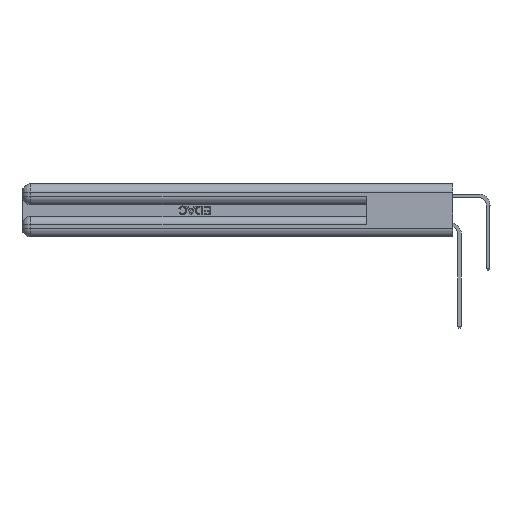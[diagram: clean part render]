
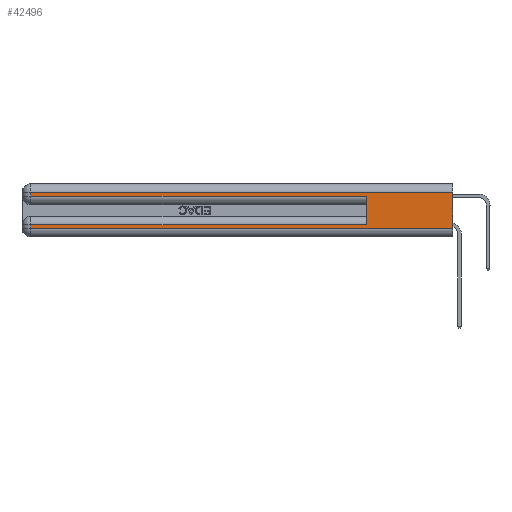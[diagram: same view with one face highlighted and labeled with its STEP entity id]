
A CAD part, left-side view. The second image highlights one B-rep face of the part: STEP entity #42496.
In plain terms, the highlighted planar face has unit normal (-1, 0, 0).
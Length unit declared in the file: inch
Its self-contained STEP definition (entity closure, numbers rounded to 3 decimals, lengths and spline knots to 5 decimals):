
#963 = LINE ( 'NONE', #32042, #27779 ) ;
#1051 = DIRECTION ( 'NONE',  ( 0., 0., -1. ) ) ;
#1064 = EDGE_CURVE ( 'NONE', #27194, #36507, #5275, .T. ) ;
#2364 = DIRECTION ( 'NONE',  ( 0., -1., 0. ) ) ;
#4359 = VERTEX_POINT ( 'NONE', #26455 ) ;
#5062 = CARTESIAN_POINT ( 'NONE',  ( 0., 2.94, 0.085 ) ) ;
#5275 = LINE ( 'NONE', #9818, #41072 ) ;
#5987 = EDGE_CURVE ( 'NONE', #21244, #41450, #963, .T. ) ;
#6390 = CARTESIAN_POINT ( 'NONE',  ( 0., 0., 0.37 ) ) ;
#7752 = VECTOR ( 'NONE', #43807, 39.37008 ) ;
#9786 = EDGE_CURVE ( 'NONE', #21244, #41560, #35603, .T. ) ;
#9818 = CARTESIAN_POINT ( 'NONE',  ( 0., 0., 0.285 ) ) ;
#12184 = ORIENTED_EDGE ( 'NONE', *, *, #14761, .T. ) ;
#12547 = VECTOR ( 'NONE', #1051, 39.37008 ) ;
#13291 = DIRECTION ( 'NONE',  ( 0., -1., 0. ) ) ;
#13956 = DIRECTION ( 'NONE',  ( 0., 0., 1. ) ) ;
#14229 = VECTOR ( 'NONE', #21004, 39.37008 ) ;
#14493 = EDGE_CURVE ( 'NONE', #41450, #27194, #43511, .T. ) ;
#14761 = EDGE_CURVE ( 'NONE', #4359, #32286, #22412, .T. ) ;
#15441 = EDGE_CURVE ( 'NONE', #32286, #34976, #23994, .T. ) ;
#15827 = ORIENTED_EDGE ( 'NONE', *, *, #40106, .T. ) ;
#16718 = DIRECTION ( 'NONE',  ( 0., 0., -1. ) ) ;
#20471 = LINE ( 'NONE', #34735, #28609 ) ;
#20824 = DIRECTION ( 'NONE',  ( 1., 0., 0. ) ) ;
#20885 = CARTESIAN_POINT ( 'NONE',  ( 0., 0.6, 0.285 ) ) ;
#21004 = DIRECTION ( 'NONE',  ( 0., 1., 0. ) ) ;
#21137 = EDGE_CURVE ( 'NONE', #4359, #36507, #20471, .T. ) ;
#21244 = VERTEX_POINT ( 'NONE', #31018 ) ;
#21519 = LINE ( 'NONE', #23303, #30763 ) ;
#21730 = CARTESIAN_POINT ( 'NONE',  ( 0., 0., 0.085 ) ) ;
#22120 = ORIENTED_EDGE ( 'NONE', *, *, #1064, .T. ) ;
#22412 = LINE ( 'NONE', #21730, #14229 ) ;
#23303 = CARTESIAN_POINT ( 'NONE',  ( 0., 0., 0.06 ) ) ;
#23689 = ORIENTED_EDGE ( 'NONE', *, *, #21137, .F. ) ;
#23994 = LINE ( 'NONE', #25380, #12547 ) ;
#25380 = CARTESIAN_POINT ( 'NONE',  ( 0., 2.94, 0.37 ) ) ;
#26134 = ORIENTED_EDGE ( 'NONE', *, *, #9786, .F. ) ;
#26455 = CARTESIAN_POINT ( 'NONE',  ( 0., 0.6, 0.085 ) ) ;
#27194 = VERTEX_POINT ( 'NONE', #33092 ) ;
#27297 = FACE_OUTER_BOUND ( 'NONE', #32736, .T. ) ;
#27779 = VECTOR ( 'NONE', #38953, 39.37008 ) ;
#28498 = AXIS2_PLACEMENT_3D ( 'NONE', #41518, #20824, #44955 ) ;
#28609 = VECTOR ( 'NONE', #13956, 39.37008 ) ;
#30123 = CARTESIAN_POINT ( 'NONE',  ( 0., 2.94, 0.37 ) ) ;
#30154 = ORIENTED_EDGE ( 'NONE', *, *, #14493, .T. ) ;
#30763 = VECTOR ( 'NONE', #2364, 39.37008 ) ;
#31018 = CARTESIAN_POINT ( 'NONE',  ( 0., 0., 0.31 ) ) ;
#31206 = CARTESIAN_POINT ( 'NONE',  ( 0., 2.94, 0.31 ) ) ;
#32042 = CARTESIAN_POINT ( 'NONE',  ( 0., 0., 0.31 ) ) ;
#32286 = VERTEX_POINT ( 'NONE', #5062 ) ;
#32736 = EDGE_LOOP ( 'NONE', ( #26134, #41705, #30154, #22120, #23689, #12184, #39008, #15827 ) ) ;
#33092 = CARTESIAN_POINT ( 'NONE',  ( 0., 2.94, 0.285 ) ) ;
#34529 = VECTOR ( 'NONE', #16718, 39.37008 ) ;
#34735 = CARTESIAN_POINT ( 'NONE',  ( 0., 0.6, 0.145 ) ) ;
#34976 = VERTEX_POINT ( 'NONE', #37746 ) ;
#35098 = CARTESIAN_POINT ( 'NONE',  ( 0., 0., 0.06 ) ) ;
#35603 = LINE ( 'NONE', #6390, #34529 ) ;
#36507 = VERTEX_POINT ( 'NONE', #20885 ) ;
#37746 = CARTESIAN_POINT ( 'NONE',  ( 0., 2.94, 0.06 ) ) ;
#38953 = DIRECTION ( 'NONE',  ( 0., 1., 0. ) ) ;
#39008 = ORIENTED_EDGE ( 'NONE', *, *, #15441, .T. ) ;
#40106 = EDGE_CURVE ( 'NONE', #34976, #41560, #21519, .T. ) ;
#41072 = VECTOR ( 'NONE', #13291, 39.37008 ) ;
#41360 = PLANE ( 'NONE',  #28498 ) ;
#41450 = VERTEX_POINT ( 'NONE', #31206 ) ;
#41518 = CARTESIAN_POINT ( 'NONE',  ( 0., 0., 0.37 ) ) ;
#41560 = VERTEX_POINT ( 'NONE', #35098 ) ;
#41705 = ORIENTED_EDGE ( 'NONE', *, *, #5987, .T. ) ;
#42496 = ADVANCED_FACE ( 'NONE', ( #27297 ), #41360, .F. ) ;
#43511 = LINE ( 'NONE', #30123, #7752 ) ;
#43807 = DIRECTION ( 'NONE',  ( 0., 0., -1. ) ) ;
#44955 = DIRECTION ( 'NONE',  ( 0., 0., -1. ) ) ;
